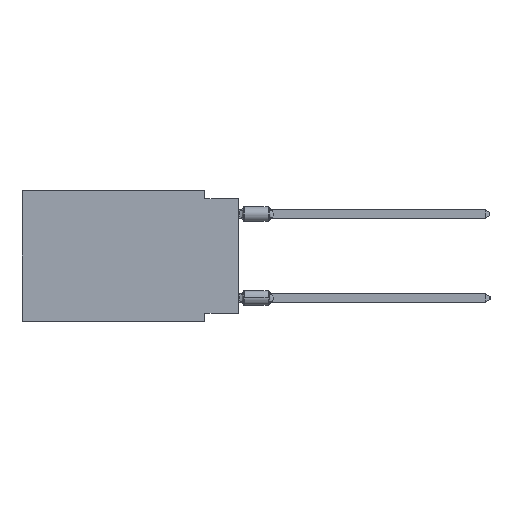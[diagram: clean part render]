
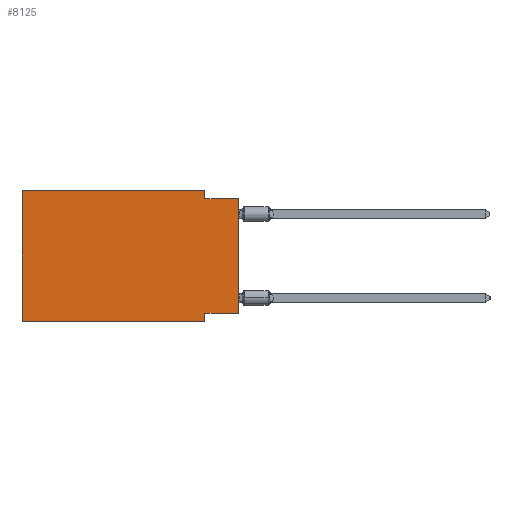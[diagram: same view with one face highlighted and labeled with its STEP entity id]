
A CAD part, left-side view. The second image highlights one B-rep face of the part: STEP entity #8125.
In plain terms, the highlighted planar face has unit normal (-1, 0, 0).
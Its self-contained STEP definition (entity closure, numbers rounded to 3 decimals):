
#101 = EDGE_CURVE ( 'NONE', #4997, #13007, #27026, .T. ) ;
#141 = ORIENTED_EDGE ( 'NONE', *, *, #101, .F. ) ;
#502 = ORIENTED_EDGE ( 'NONE', *, *, #13282, .F. ) ;
#608 = VERTEX_POINT ( 'NONE', #7818 ) ;
#924 = DIRECTION ( 'NONE',  ( 1., 0., 0. ) ) ;
#1117 = DIRECTION ( 'NONE',  ( 0., 0., -1. ) ) ;
#3721 = PLANE ( 'NONE',  #22297 ) ;
#4997 = VERTEX_POINT ( 'NONE', #36646 ) ;
#5841 = VECTOR ( 'NONE', #17419, 1000. ) ;
#5877 = LINE ( 'NONE', #14257, #5841 ) ;
#5959 = EDGE_CURVE ( 'NONE', #34313, #13007, #28737, .T. ) ;
#6019 = FACE_OUTER_BOUND ( 'NONE', #24912, .T. ) ;
#6672 = VECTOR ( 'NONE', #32814, 1000. ) ;
#7818 = CARTESIAN_POINT ( 'NONE',  ( 0., 0., -9.271 ) ) ;
#8125 = ADVANCED_FACE ( 'NONE', ( #6019 ), #3721, .F. ) ;
#9398 = LINE ( 'NONE', #17791, #34271 ) ;
#10340 = DIRECTION ( 'NONE',  ( 0., 0., -1. ) ) ;
#11001 = CARTESIAN_POINT ( 'NONE',  ( 0., 0., -0.635 ) ) ;
#11371 = ORIENTED_EDGE ( 'NONE', *, *, #21815, .F. ) ;
#11889 = CARTESIAN_POINT ( 'NONE',  ( 0., 2.54, -9.906 ) ) ;
#12379 = EDGE_CURVE ( 'NONE', #608, #4997, #9398, .T. ) ;
#12548 = DIRECTION ( 'NONE',  ( 0., 1., 0. ) ) ;
#13007 = VERTEX_POINT ( 'NONE', #11889 ) ;
#13078 = CARTESIAN_POINT ( 'NONE',  ( 0., 2.54, -9.906 ) ) ;
#13098 = ORIENTED_EDGE ( 'NONE', *, *, #17800, .T. ) ;
#13260 = LINE ( 'NONE', #31524, #32531 ) ;
#13282 = EDGE_CURVE ( 'NONE', #26287, #18826, #33816, .T. ) ;
#14257 = CARTESIAN_POINT ( 'NONE',  ( 0., 0., 0. ) ) ;
#14365 = EDGE_CURVE ( 'NONE', #18826, #34641, #36507, .T. ) ;
#14722 = VECTOR ( 'NONE', #10340, 1000. ) ;
#17010 = CARTESIAN_POINT ( 'NONE',  ( 0., 16.383, -9.906 ) ) ;
#17419 = DIRECTION ( 'NONE',  ( 0., 0., 1. ) ) ;
#17791 = CARTESIAN_POINT ( 'NONE',  ( 0., 0., -9.271 ) ) ;
#17800 = EDGE_CURVE ( 'NONE', #608, #34641, #5877, .T. ) ;
#18654 = CARTESIAN_POINT ( 'NONE',  ( 0., 2.54, 0. ) ) ;
#18826 = VERTEX_POINT ( 'NONE', #25706 ) ;
#18974 = VECTOR ( 'NONE', #20192, 1000. ) ;
#19959 = LINE ( 'NONE', #31682, #24405 ) ;
#20192 = DIRECTION ( 'NONE',  ( 0., -1., 0. ) ) ;
#20329 = CARTESIAN_POINT ( 'NONE',  ( 0., 0., -0.635 ) ) ;
#21815 = EDGE_CURVE ( 'NONE', #34313, #31299, #19959, .T. ) ;
#21961 = ORIENTED_EDGE ( 'NONE', *, *, #5959, .T. ) ;
#22297 = AXIS2_PLACEMENT_3D ( 'NONE', #26417, #924, #1117 ) ;
#23040 = ORIENTED_EDGE ( 'NONE', *, *, #12379, .F. ) ;
#24405 = VECTOR ( 'NONE', #28888, 1000. ) ;
#24912 = EDGE_LOOP ( 'NONE', ( #13098, #35274, #502, #27815, #11371, #21961, #141, #23040 ) ) ;
#25219 = CARTESIAN_POINT ( 'NONE',  ( 0., 2.54, 0. ) ) ;
#25544 = DIRECTION ( 'NONE',  ( 0., -1., 0. ) ) ;
#25706 = CARTESIAN_POINT ( 'NONE',  ( 0., 2.54, -0.635 ) ) ;
#26287 = VERTEX_POINT ( 'NONE', #18654 ) ;
#26417 = CARTESIAN_POINT ( 'NONE',  ( 0., 16.383, 0. ) ) ;
#27026 = LINE ( 'NONE', #13078, #6672 ) ;
#27815 = ORIENTED_EDGE ( 'NONE', *, *, #34205, .F. ) ;
#28737 = LINE ( 'NONE', #17010, #18974 ) ;
#28888 = DIRECTION ( 'NONE',  ( 0., 0., 1. ) ) ;
#31299 = VERTEX_POINT ( 'NONE', #36006 ) ;
#31524 = CARTESIAN_POINT ( 'NONE',  ( 0., 16.383, 0. ) ) ;
#31682 = CARTESIAN_POINT ( 'NONE',  ( 0., 16.383, 0. ) ) ;
#32531 = VECTOR ( 'NONE', #25544, 1000. ) ;
#32814 = DIRECTION ( 'NONE',  ( 0., 0., -1. ) ) ;
#33432 = VECTOR ( 'NONE', #33722, 1000. ) ;
#33722 = DIRECTION ( 'NONE',  ( 0., -1., 0. ) ) ;
#33816 = LINE ( 'NONE', #25219, #14722 ) ;
#34205 = EDGE_CURVE ( 'NONE', #31299, #26287, #13260, .T. ) ;
#34271 = VECTOR ( 'NONE', #12548, 1000. ) ;
#34313 = VERTEX_POINT ( 'NONE', #34741 ) ;
#34641 = VERTEX_POINT ( 'NONE', #20329 ) ;
#34741 = CARTESIAN_POINT ( 'NONE',  ( 0., 16.383, -9.906 ) ) ;
#35274 = ORIENTED_EDGE ( 'NONE', *, *, #14365, .F. ) ;
#36006 = CARTESIAN_POINT ( 'NONE',  ( 0., 16.383, 0. ) ) ;
#36507 = LINE ( 'NONE', #11001, #33432 ) ;
#36646 = CARTESIAN_POINT ( 'NONE',  ( 0., 2.54, -9.271 ) ) ;
